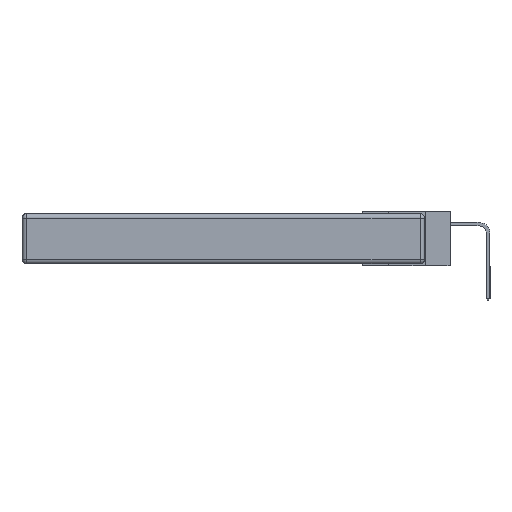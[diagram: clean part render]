
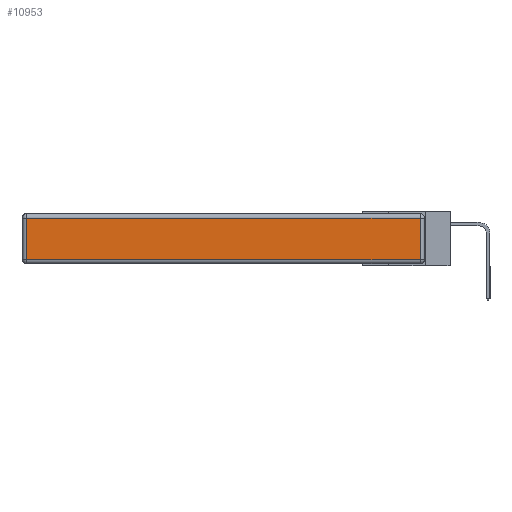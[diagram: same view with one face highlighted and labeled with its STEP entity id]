
A CAD part, left-side view. The second image highlights one B-rep face of the part: STEP entity #10953.
In plain terms, the highlighted planar face has unit normal (-1, 0, 0).
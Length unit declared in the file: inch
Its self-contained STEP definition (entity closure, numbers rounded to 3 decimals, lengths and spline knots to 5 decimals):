
#486 = LINE ( 'NONE', #9451, #3882 ) ;
#732 = EDGE_CURVE ( 'NONE', #8450, #6088, #486, .T. ) ;
#2079 = PLANE ( 'NONE',  #16597 ) ;
#2197 = DIRECTION ( 'NONE',  ( -1., 0., 0. ) ) ;
#2273 = EDGE_CURVE ( 'NONE', #13134, #8450, #16818, .T. ) ;
#2936 = CARTESIAN_POINT ( 'NONE',  ( 0., 2.72, -0.343 ) ) ;
#3464 = CARTESIAN_POINT ( 'NONE',  ( 0., 0., -0.343 ) ) ;
#3882 = VECTOR ( 'NONE', #16286, 39.37008 ) ;
#4810 = EDGE_CURVE ( 'NONE', #10132, #13134, #9418, .T. ) ;
#4899 = ORIENTED_EDGE ( 'NONE', *, *, #2273, .T. ) ;
#5387 = DIRECTION ( 'NONE',  ( 0., 0., 1. ) ) ;
#5506 = DIRECTION ( 'NONE',  ( 0., 0., -1. ) ) ;
#6088 = VERTEX_POINT ( 'NONE', #15537 ) ;
#6643 = VECTOR ( 'NONE', #13912, 39.37008 ) ;
#6684 = FACE_OUTER_BOUND ( 'NONE', #7829, .T. ) ;
#7152 = ORIENTED_EDGE ( 'NONE', *, *, #4810, .T. ) ;
#7829 = EDGE_LOOP ( 'NONE', ( #12655, #11809, #7152, #4899 ) ) ;
#8450 = VERTEX_POINT ( 'NONE', #11061 ) ;
#8670 = CARTESIAN_POINT ( 'NONE',  ( 0., 2.75, -0.03 ) ) ;
#9418 = LINE ( 'NONE', #8670, #6643 ) ;
#9451 = CARTESIAN_POINT ( 'NONE',  ( 0., 0., -0.313 ) ) ;
#9489 = VECTOR ( 'NONE', #5387, 39.37008 ) ;
#10132 = VERTEX_POINT ( 'NONE', #17003 ) ;
#10646 = CARTESIAN_POINT ( 'NONE',  ( 0., 0.03, -0.343 ) ) ;
#10953 = ADVANCED_FACE ( 'NONE', ( #6684 ), #2079, .T. ) ;
#11061 = CARTESIAN_POINT ( 'NONE',  ( 0., 2.72, -0.313 ) ) ;
#11809 = ORIENTED_EDGE ( 'NONE', *, *, #17109, .T. ) ;
#12161 = CARTESIAN_POINT ( 'NONE',  ( 0., 2.72, -0.03 ) ) ;
#12655 = ORIENTED_EDGE ( 'NONE', *, *, #732, .T. ) ;
#13109 = LINE ( 'NONE', #10646, #9489 ) ;
#13134 = VERTEX_POINT ( 'NONE', #12161 ) ;
#13912 = DIRECTION ( 'NONE',  ( 0., 1., 0. ) ) ;
#15320 = VECTOR ( 'NONE', #5506, 39.37008 ) ;
#15537 = CARTESIAN_POINT ( 'NONE',  ( 0., 0.03, -0.313 ) ) ;
#16182 = DIRECTION ( 'NONE',  ( 0., 0., 1. ) ) ;
#16286 = DIRECTION ( 'NONE',  ( 0., -1., 0. ) ) ;
#16597 = AXIS2_PLACEMENT_3D ( 'NONE', #3464, #2197, #16182 ) ;
#16818 = LINE ( 'NONE', #2936, #15320 ) ;
#17003 = CARTESIAN_POINT ( 'NONE',  ( 0., 0.03, -0.03 ) ) ;
#17109 = EDGE_CURVE ( 'NONE', #6088, #10132, #13109, .T. ) ;
